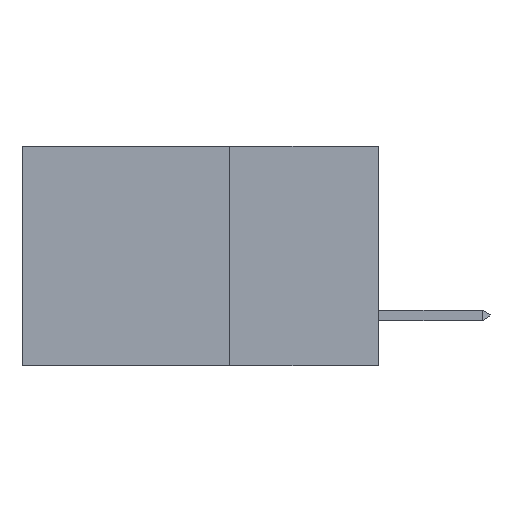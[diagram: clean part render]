
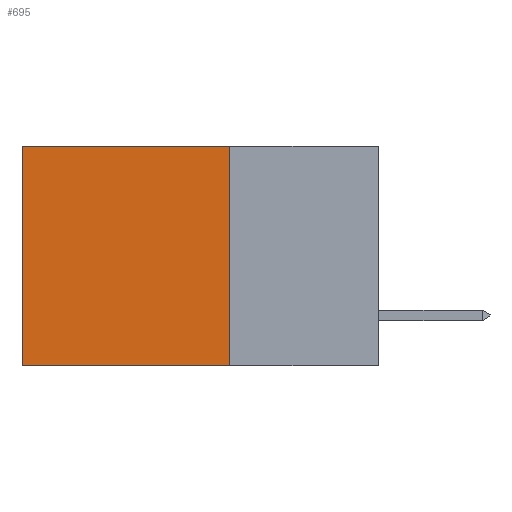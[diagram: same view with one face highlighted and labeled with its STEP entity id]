
A CAD part, left-side view. The second image highlights one B-rep face of the part: STEP entity #695.
In plain terms, the highlighted planar face has unit normal (-1, 0, 0).
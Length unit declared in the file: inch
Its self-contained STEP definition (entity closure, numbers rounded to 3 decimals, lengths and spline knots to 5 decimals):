
#695 = ADVANCED_FACE ( 'NONE', ( #15281 ), #18514, .F. ) ;
#1906 = VERTEX_POINT ( 'NONE', #4970 ) ;
#3645 = VECTOR ( 'NONE', #17614, 39.37008 ) ;
#3722 = CARTESIAN_POINT ( 'NONE',  ( 0.2615, 0.25, 0. ) ) ;
#4066 = LINE ( 'NONE', #18722, #18875 ) ;
#4572 = EDGE_CURVE ( 'NONE', #1906, #4997, #17944, .T. ) ;
#4970 = CARTESIAN_POINT ( 'NONE',  ( 0.2615, 0.25, 0. ) ) ;
#4997 = VERTEX_POINT ( 'NONE', #9678 ) ;
#5193 = VECTOR ( 'NONE', #13272, 39.37008 ) ;
#5294 = CARTESIAN_POINT ( 'NONE',  ( 0.2615, 0.25, -0.37 ) ) ;
#5620 = VERTEX_POINT ( 'NONE', #11893 ) ;
#7491 = ORIENTED_EDGE ( 'NONE', *, *, #9421, .T. ) ;
#8869 = DIRECTION ( 'NONE',  ( 0., 0., -1. ) ) ;
#9164 = CARTESIAN_POINT ( 'NONE',  ( 0.2615, 0.25, -0.37 ) ) ;
#9421 = EDGE_CURVE ( 'NONE', #19234, #5620, #4066, .T. ) ;
#9678 = CARTESIAN_POINT ( 'NONE',  ( 0.2615, 0.25, -0.37 ) ) ;
#9905 = EDGE_CURVE ( 'NONE', #4997, #5620, #14011, .T. ) ;
#11893 = CARTESIAN_POINT ( 'NONE',  ( 0.2615, 0.6, -0.37 ) ) ;
#12838 = CARTESIAN_POINT ( 'NONE',  ( 0.2615, 0.25, -0.37 ) ) ;
#13272 = DIRECTION ( 'NONE',  ( 0., 1., 0. ) ) ;
#13914 = EDGE_LOOP ( 'NONE', ( #7491, #20920, #20522, #18996 ) ) ;
#14011 = LINE ( 'NONE', #9164, #3645 ) ;
#14304 = CARTESIAN_POINT ( 'NONE',  ( 0.2615, 0.6, 0. ) ) ;
#15137 = EDGE_CURVE ( 'NONE', #1906, #19234, #18700, .T. ) ;
#15281 = FACE_OUTER_BOUND ( 'NONE', #13914, .T. ) ;
#16530 = VECTOR ( 'NONE', #19454, 39.37008 ) ;
#16577 = AXIS2_PLACEMENT_3D ( 'NONE', #5294, #16672, #16896 ) ;
#16672 = DIRECTION ( 'NONE',  ( 1., 0., 0. ) ) ;
#16896 = DIRECTION ( 'NONE',  ( 0., 0., -1. ) ) ;
#17614 = DIRECTION ( 'NONE',  ( 0., 1., 0. ) ) ;
#17944 = LINE ( 'NONE', #12838, #16530 ) ;
#18514 = PLANE ( 'NONE',  #16577 ) ;
#18700 = LINE ( 'NONE', #3722, #5193 ) ;
#18722 = CARTESIAN_POINT ( 'NONE',  ( 0.2615, 0.6, -0.37 ) ) ;
#18875 = VECTOR ( 'NONE', #8869, 39.37008 ) ;
#18996 = ORIENTED_EDGE ( 'NONE', *, *, #15137, .T. ) ;
#19234 = VERTEX_POINT ( 'NONE', #14304 ) ;
#19454 = DIRECTION ( 'NONE',  ( 0., 0., -1. ) ) ;
#20522 = ORIENTED_EDGE ( 'NONE', *, *, #4572, .F. ) ;
#20920 = ORIENTED_EDGE ( 'NONE', *, *, #9905, .F. ) ;
